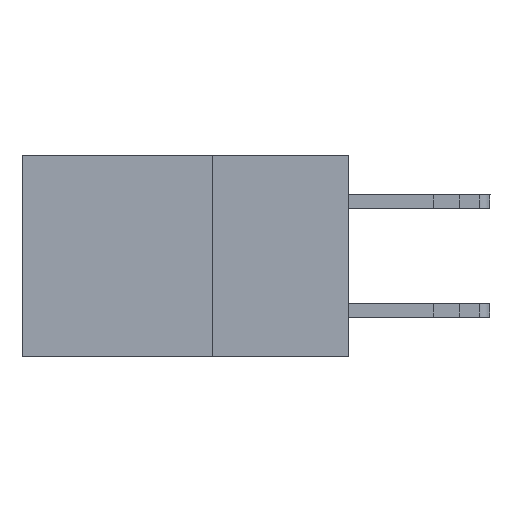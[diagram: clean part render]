
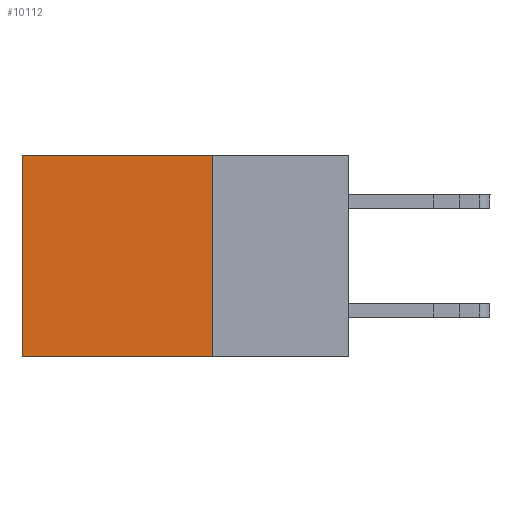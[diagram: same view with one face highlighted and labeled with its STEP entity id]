
A CAD part, left-side view. The second image highlights one B-rep face of the part: STEP entity #10112.
In plain terms, the highlighted planar face has unit normal (-1, 0, 0).
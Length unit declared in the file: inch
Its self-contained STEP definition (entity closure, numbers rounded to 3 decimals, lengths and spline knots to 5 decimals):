
#366 = VECTOR ( 'NONE', #8414, 39.37008 ) ;
#875 = DIRECTION ( 'NONE',  ( 0., 0., -1. ) ) ;
#1211 = ORIENTED_EDGE ( 'NONE', *, *, #10009, .F. ) ;
#2456 = VECTOR ( 'NONE', #6869, 39.37008 ) ;
#2513 = CARTESIAN_POINT ( 'NONE',  ( 0.298, 0.25, 0. ) ) ;
#2966 = VERTEX_POINT ( 'NONE', #12120 ) ;
#3869 = PLANE ( 'NONE',  #9141 ) ;
#3877 = VECTOR ( 'NONE', #16713, 39.37008 ) ;
#4778 = EDGE_CURVE ( 'NONE', #2966, #10024, #13627, .T. ) ;
#4906 = DIRECTION ( 'NONE',  ( 0., 0., -1. ) ) ;
#6109 = ORIENTED_EDGE ( 'NONE', *, *, #4778, .F. ) ;
#6869 = DIRECTION ( 'NONE',  ( 0., 1., 0. ) ) ;
#7463 = LINE ( 'NONE', #10208, #16215 ) ;
#8414 = DIRECTION ( 'NONE',  ( 0., 1., 0. ) ) ;
#8917 = ORIENTED_EDGE ( 'NONE', *, *, #13072, .T. ) ;
#9096 = CARTESIAN_POINT ( 'NONE',  ( 0.298, 0.25, 0. ) ) ;
#9141 = AXIS2_PLACEMENT_3D ( 'NONE', #9096, #12611, #875 ) ;
#9957 = CARTESIAN_POINT ( 'NONE',  ( 0.298, 0.25, 0. ) ) ;
#10009 = EDGE_CURVE ( 'NONE', #16607, #2966, #7463, .T. ) ;
#10024 = VERTEX_POINT ( 'NONE', #11496 ) ;
#10112 = ADVANCED_FACE ( 'NONE', ( #11672 ), #3869, .F. ) ;
#10208 = CARTESIAN_POINT ( 'NONE',  ( 0.298, 0.25, 0. ) ) ;
#10231 = ORIENTED_EDGE ( 'NONE', *, *, #11131, .T. ) ;
#10865 = VERTEX_POINT ( 'NONE', #15273 ) ;
#11131 = EDGE_CURVE ( 'NONE', #16607, #10865, #13800, .T. ) ;
#11163 = LINE ( 'NONE', #16372, #3877 ) ;
#11496 = CARTESIAN_POINT ( 'NONE',  ( 0.298, 0.6, -0.37 ) ) ;
#11672 = FACE_OUTER_BOUND ( 'NONE', #15517, .T. ) ;
#12120 = CARTESIAN_POINT ( 'NONE',  ( 0.298, 0.25, -0.37 ) ) ;
#12363 = CARTESIAN_POINT ( 'NONE',  ( 0.298, 0.25, -0.37 ) ) ;
#12611 = DIRECTION ( 'NONE',  ( 1., 0., 0. ) ) ;
#13072 = EDGE_CURVE ( 'NONE', #10865, #10024, #11163, .T. ) ;
#13627 = LINE ( 'NONE', #12363, #2456 ) ;
#13800 = LINE ( 'NONE', #9957, #366 ) ;
#15273 = CARTESIAN_POINT ( 'NONE',  ( 0.298, 0.6, 0. ) ) ;
#15517 = EDGE_LOOP ( 'NONE', ( #8917, #6109, #1211, #10231 ) ) ;
#16215 = VECTOR ( 'NONE', #4906, 39.37008 ) ;
#16372 = CARTESIAN_POINT ( 'NONE',  ( 0.298, 0.6, 0. ) ) ;
#16607 = VERTEX_POINT ( 'NONE', #2513 ) ;
#16713 = DIRECTION ( 'NONE',  ( 0., 0., -1. ) ) ;
